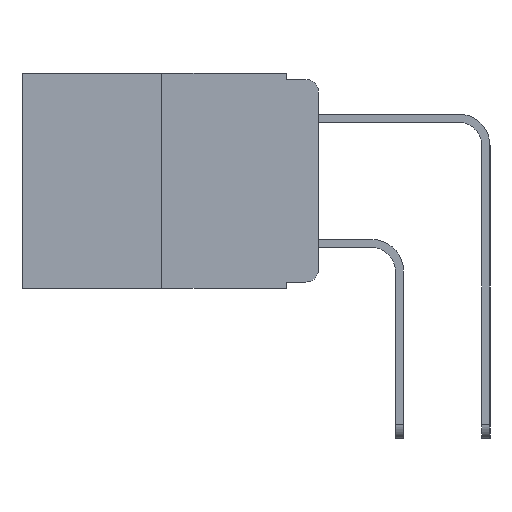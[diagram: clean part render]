
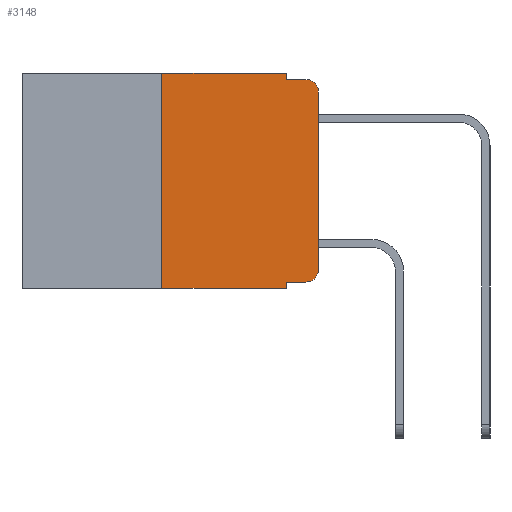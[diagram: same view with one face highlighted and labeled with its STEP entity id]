
A CAD part, left-side view. The second image highlights one B-rep face of the part: STEP entity #3148.
In plain terms, the highlighted planar face has unit normal (-1, 0, 0).
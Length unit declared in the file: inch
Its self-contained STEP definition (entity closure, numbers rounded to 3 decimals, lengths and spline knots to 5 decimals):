
#290 = CARTESIAN_POINT ( 'NONE',  ( 0., 0.02, -0.333 ) ) ;
#301 = DIRECTION ( 'NONE',  ( 0., -1., 0. ) ) ;
#523 = CARTESIAN_POINT ( 'NONE',  ( 0., 0.051, 0. ) ) ;
#806 = ORIENTED_EDGE ( 'NONE', *, *, #6493, .T. ) ;
#858 = VERTEX_POINT ( 'NONE', #290 ) ;
#1269 = CARTESIAN_POINT ( 'NONE',  ( 0., 0., -0.313 ) ) ;
#1544 = ORIENTED_EDGE ( 'NONE', *, *, #5813, .F. ) ;
#1604 = CARTESIAN_POINT ( 'NONE',  ( 0., 0., -0.03 ) ) ;
#1786 = DIRECTION ( 'NONE',  ( 1., 0., 0. ) ) ;
#1823 = VECTOR ( 'NONE', #6587, 39.37008 ) ;
#1873 = CIRCLE ( 'NONE', #2716, 0.02 ) ;
#2012 = LINE ( 'NONE', #7456, #12631 ) ;
#2415 = CARTESIAN_POINT ( 'NONE',  ( 0., 0.02, -0.03 ) ) ;
#2416 = CARTESIAN_POINT ( 'NONE',  ( 0., 0.473, 0. ) ) ;
#2428 = VERTEX_POINT ( 'NONE', #1604 ) ;
#2453 = VECTOR ( 'NONE', #8662, 39.37008 ) ;
#2670 = EDGE_CURVE ( 'NONE', #4630, #4740, #8054, .T. ) ;
#2716 = AXIS2_PLACEMENT_3D ( 'NONE', #2415, #9434, #3446 ) ;
#3113 = EDGE_CURVE ( 'NONE', #12129, #5133, #12943, .T. ) ;
#3148 = ADVANCED_FACE ( 'NONE', ( #12641 ), #12319, .F. ) ;
#3446 = DIRECTION ( 'NONE',  ( 0., 0., -1. ) ) ;
#3461 = ORIENTED_EDGE ( 'NONE', *, *, #3113, .F. ) ;
#3577 = ORIENTED_EDGE ( 'NONE', *, *, #12271, .T. ) ;
#3859 = DIRECTION ( 'NONE',  ( 0., 0., -1. ) ) ;
#4018 = CARTESIAN_POINT ( 'NONE',  ( 0., 0.051, 0. ) ) ;
#4187 = CARTESIAN_POINT ( 'NONE',  ( 0., 0.473, 0. ) ) ;
#4193 = VECTOR ( 'NONE', #11982, 39.37008 ) ;
#4194 = VERTEX_POINT ( 'NONE', #7594 ) ;
#4222 = CARTESIAN_POINT ( 'NONE',  ( 0., 0.051, -0.01 ) ) ;
#4426 = ORIENTED_EDGE ( 'NONE', *, *, #12923, .T. ) ;
#4630 = VERTEX_POINT ( 'NONE', #5070 ) ;
#4692 = EDGE_CURVE ( 'NONE', #4194, #12129, #7225, .T. ) ;
#4740 = VERTEX_POINT ( 'NONE', #10819 ) ;
#5004 = VERTEX_POINT ( 'NONE', #1269 ) ;
#5014 = DIRECTION ( 'NONE',  ( -1., 0., 0. ) ) ;
#5070 = CARTESIAN_POINT ( 'NONE',  ( 0., 0.051, -0.333 ) ) ;
#5133 = VERTEX_POINT ( 'NONE', #4018 ) ;
#5488 = ORIENTED_EDGE ( 'NONE', *, *, #11298, .T. ) ;
#5813 = EDGE_CURVE ( 'NONE', #9628, #7400, #9880, .T. ) ;
#5942 = CARTESIAN_POINT ( 'NONE',  ( 0., 0.02, -0.01 ) ) ;
#6493 = EDGE_CURVE ( 'NONE', #2428, #7400, #1873, .T. ) ;
#6587 = DIRECTION ( 'NONE',  ( 0., 0., 1. ) ) ;
#6745 = ORIENTED_EDGE ( 'NONE', *, *, #2670, .F. ) ;
#6806 = ORIENTED_EDGE ( 'NONE', *, *, #12681, .F. ) ;
#6853 = CARTESIAN_POINT ( 'NONE',  ( 0., 0.051, -0.01 ) ) ;
#7225 = LINE ( 'NONE', #11407, #1823 ) ;
#7353 = VECTOR ( 'NONE', #8079, 39.37008 ) ;
#7400 = VERTEX_POINT ( 'NONE', #5942 ) ;
#7456 = CARTESIAN_POINT ( 'NONE',  ( 0., 0.473, -0.343 ) ) ;
#7594 = CARTESIAN_POINT ( 'NONE',  ( 0., 0.25, -0.343 ) ) ;
#7696 = CARTESIAN_POINT ( 'NONE',  ( 0., 0.051, 0. ) ) ;
#7731 = VECTOR ( 'NONE', #9985, 39.37008 ) ;
#7839 = LINE ( 'NONE', #523, #2453 ) ;
#8054 = LINE ( 'NONE', #7696, #9733 ) ;
#8079 = DIRECTION ( 'NONE',  ( 0., -1., 0. ) ) ;
#8105 = ORIENTED_EDGE ( 'NONE', *, *, #4692, .F. ) ;
#8662 = DIRECTION ( 'NONE',  ( 0., 0., -1. ) ) ;
#9031 = CARTESIAN_POINT ( 'NONE',  ( 0., 0., 0. ) ) ;
#9089 = AXIS2_PLACEMENT_3D ( 'NONE', #2416, #1786, #3859 ) ;
#9158 = EDGE_CURVE ( 'NONE', #5004, #2428, #12419, .T. ) ;
#9434 = DIRECTION ( 'NONE',  ( -1., 0., 0. ) ) ;
#9573 = VECTOR ( 'NONE', #11667, 39.37008 ) ;
#9628 = VERTEX_POINT ( 'NONE', #6853 ) ;
#9733 = VECTOR ( 'NONE', #12897, 39.37008 ) ;
#9778 = ORIENTED_EDGE ( 'NONE', *, *, #9158, .T. ) ;
#9880 = LINE ( 'NONE', #4222, #9573 ) ;
#9975 = LINE ( 'NONE', #12000, #7353 ) ;
#9985 = DIRECTION ( 'NONE',  ( 0., -1., 0. ) ) ;
#10713 = CARTESIAN_POINT ( 'NONE',  ( 0., 0.25, 0. ) ) ;
#10819 = CARTESIAN_POINT ( 'NONE',  ( 0., 0.051, -0.343 ) ) ;
#10980 = CARTESIAN_POINT ( 'NONE',  ( 0., 0.02, -0.313 ) ) ;
#11185 = EDGE_LOOP ( 'NONE', ( #9778, #806, #1544, #6806, #3461, #8105, #5488, #6745, #4426, #3577 ) ) ;
#11298 = EDGE_CURVE ( 'NONE', #4194, #4740, #2012, .T. ) ;
#11407 = CARTESIAN_POINT ( 'NONE',  ( 0., 0.25, 0. ) ) ;
#11410 = AXIS2_PLACEMENT_3D ( 'NONE', #10980, #5014, #11970 ) ;
#11667 = DIRECTION ( 'NONE',  ( 0., -1., 0. ) ) ;
#11970 = DIRECTION ( 'NONE',  ( 0., 0., -1. ) ) ;
#11982 = DIRECTION ( 'NONE',  ( 0., 0., 1. ) ) ;
#12000 = CARTESIAN_POINT ( 'NONE',  ( 0., 0.051, -0.333 ) ) ;
#12129 = VERTEX_POINT ( 'NONE', #10713 ) ;
#12271 = EDGE_CURVE ( 'NONE', #858, #5004, #12446, .T. ) ;
#12319 = PLANE ( 'NONE',  #9089 ) ;
#12419 = LINE ( 'NONE', #9031, #4193 ) ;
#12446 = CIRCLE ( 'NONE', #11410, 0.02 ) ;
#12631 = VECTOR ( 'NONE', #301, 39.37008 ) ;
#12641 = FACE_OUTER_BOUND ( 'NONE', #11185, .T. ) ;
#12681 = EDGE_CURVE ( 'NONE', #5133, #9628, #7839, .T. ) ;
#12897 = DIRECTION ( 'NONE',  ( 0., 0., -1. ) ) ;
#12923 = EDGE_CURVE ( 'NONE', #4630, #858, #9975, .T. ) ;
#12943 = LINE ( 'NONE', #4187, #7731 ) ;
